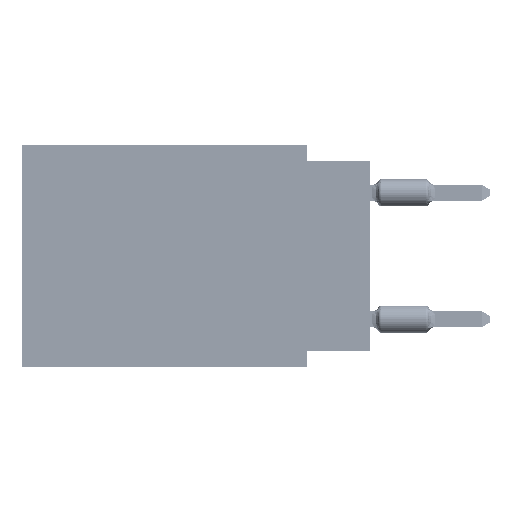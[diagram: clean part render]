
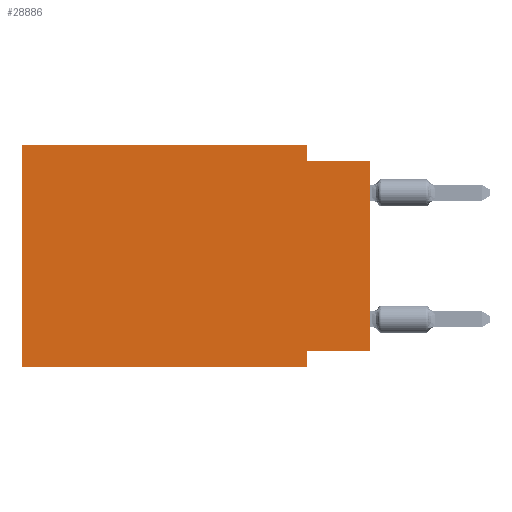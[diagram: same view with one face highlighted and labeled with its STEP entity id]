
A CAD part, left-side view. The second image highlights one B-rep face of the part: STEP entity #28886.
In plain terms, the highlighted planar face has unit normal (-1, 0, 0).
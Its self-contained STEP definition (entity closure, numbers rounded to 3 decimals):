
#2972 = EDGE_CURVE ( 'NONE', #65100, #48539, #5425, .T. ) ;
#3996 = PLANE ( 'NONE',  #25015 ) ;
#4470 = EDGE_CURVE ( 'NONE', #5256, #47302, #30722, .T. ) ;
#5256 = VERTEX_POINT ( 'NONE', #74666 ) ;
#5425 = LINE ( 'NONE', #38827, #81942 ) ;
#5709 = ORIENTED_EDGE ( 'NONE', *, *, #71002, .F. ) ;
#6397 = DIRECTION ( 'NONE',  ( 0., 1., 0. ) ) ;
#9095 = ORIENTED_EDGE ( 'NONE', *, *, #2972, .F. ) ;
#10386 = LINE ( 'NONE', #25479, #15907 ) ;
#15907 = VECTOR ( 'NONE', #17061, 1000. ) ;
#17061 = DIRECTION ( 'NONE',  ( 0., 0., 1. ) ) ;
#18323 = CARTESIAN_POINT ( 'NONE',  ( 0., 0., -8.255 ) ) ;
#18879 = CARTESIAN_POINT ( 'NONE',  ( 0., 0., -8.255 ) ) ;
#20419 = CARTESIAN_POINT ( 'NONE',  ( 0., 13.97, 0. ) ) ;
#21576 = VERTEX_POINT ( 'NONE', #40463 ) ;
#21836 = VECTOR ( 'NONE', #61711, 1000. ) ;
#23584 = FACE_OUTER_BOUND ( 'NONE', #56239, .T. ) ;
#24513 = VERTEX_POINT ( 'NONE', #36314 ) ;
#25015 = AXIS2_PLACEMENT_3D ( 'NONE', #44948, #64988, #50738 ) ;
#25479 = CARTESIAN_POINT ( 'NONE',  ( 0., 0., 0. ) ) ;
#25960 = VERTEX_POINT ( 'NONE', #84223 ) ;
#26146 = ORIENTED_EDGE ( 'NONE', *, *, #66307, .T. ) ;
#27733 = EDGE_CURVE ( 'NONE', #25960, #24513, #73412, .T. ) ;
#28886 = ADVANCED_FACE ( 'NONE', ( #23584 ), #3996, .F. ) ;
#30722 = LINE ( 'NONE', #49454, #49456 ) ;
#30952 = VERTEX_POINT ( 'NONE', #18323 ) ;
#31157 = CARTESIAN_POINT ( 'NONE',  ( 0., 2.54, -0.635 ) ) ;
#32793 = ORIENTED_EDGE ( 'NONE', *, *, #27733, .F. ) ;
#34018 = VECTOR ( 'NONE', #6397, 1000. ) ;
#34550 = LINE ( 'NONE', #49971, #21836 ) ;
#35477 = ORIENTED_EDGE ( 'NONE', *, *, #76413, .T. ) ;
#36314 = CARTESIAN_POINT ( 'NONE',  ( 0., 13.97, 0. ) ) ;
#38827 = CARTESIAN_POINT ( 'NONE',  ( 0., 2.54, -8.89 ) ) ;
#39130 = DIRECTION ( 'NONE',  ( 0., 0., 1. ) ) ;
#40463 = CARTESIAN_POINT ( 'NONE',  ( 0., 0., -0.635 ) ) ;
#42504 = LINE ( 'NONE', #62976, #60685 ) ;
#43017 = DIRECTION ( 'NONE',  ( 0., -1., 0. ) ) ;
#44948 = CARTESIAN_POINT ( 'NONE',  ( 0., 13.97, 0. ) ) ;
#47302 = VERTEX_POINT ( 'NONE', #31157 ) ;
#47886 = EDGE_CURVE ( 'NONE', #30952, #65100, #66930, .T. ) ;
#48539 = VERTEX_POINT ( 'NONE', #84579 ) ;
#49454 = CARTESIAN_POINT ( 'NONE',  ( 0., 2.54, 0. ) ) ;
#49456 = VECTOR ( 'NONE', #77918, 1000. ) ;
#49971 = CARTESIAN_POINT ( 'NONE',  ( 0., 13.97, -8.89 ) ) ;
#50123 = CARTESIAN_POINT ( 'NONE',  ( 0., 2.54, -8.255 ) ) ;
#50713 = ORIENTED_EDGE ( 'NONE', *, *, #4470, .F. ) ;
#50738 = DIRECTION ( 'NONE',  ( 0., 0., -1. ) ) ;
#56239 = EDGE_LOOP ( 'NONE', ( #26146, #5709, #50713, #86274, #32793, #35477, #9095, #78933 ) ) ;
#59739 = DIRECTION ( 'NONE',  ( 0., 0., -1. ) ) ;
#60685 = VECTOR ( 'NONE', #75470, 1000. ) ;
#61711 = DIRECTION ( 'NONE',  ( 0., -1., 0. ) ) ;
#62976 = CARTESIAN_POINT ( 'NONE',  ( 0., 13.97, 0. ) ) ;
#63274 = VECTOR ( 'NONE', #39130, 1000. ) ;
#63919 = CARTESIAN_POINT ( 'NONE',  ( 0., 0., -0.635 ) ) ;
#64988 = DIRECTION ( 'NONE',  ( 1., 0., 0. ) ) ;
#65100 = VERTEX_POINT ( 'NONE', #50123 ) ;
#66307 = EDGE_CURVE ( 'NONE', #30952, #21576, #10386, .T. ) ;
#66831 = VECTOR ( 'NONE', #43017, 1000. ) ;
#66930 = LINE ( 'NONE', #18879, #34018 ) ;
#71002 = EDGE_CURVE ( 'NONE', #47302, #21576, #83963, .T. ) ;
#73412 = LINE ( 'NONE', #20419, #63274 ) ;
#74666 = CARTESIAN_POINT ( 'NONE',  ( 0., 2.54, 0. ) ) ;
#75470 = DIRECTION ( 'NONE',  ( 0., -1., 0. ) ) ;
#76413 = EDGE_CURVE ( 'NONE', #25960, #48539, #34550, .T. ) ;
#77918 = DIRECTION ( 'NONE',  ( 0., 0., -1. ) ) ;
#78933 = ORIENTED_EDGE ( 'NONE', *, *, #47886, .F. ) ;
#81942 = VECTOR ( 'NONE', #59739, 1000. ) ;
#83468 = EDGE_CURVE ( 'NONE', #24513, #5256, #42504, .T. ) ;
#83963 = LINE ( 'NONE', #63919, #66831 ) ;
#84223 = CARTESIAN_POINT ( 'NONE',  ( 0., 13.97, -8.89 ) ) ;
#84579 = CARTESIAN_POINT ( 'NONE',  ( 0., 2.54, -8.89 ) ) ;
#86274 = ORIENTED_EDGE ( 'NONE', *, *, #83468, .F. ) ;
